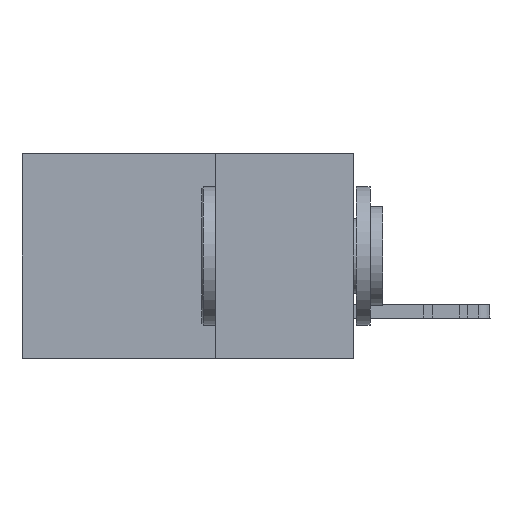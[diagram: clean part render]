
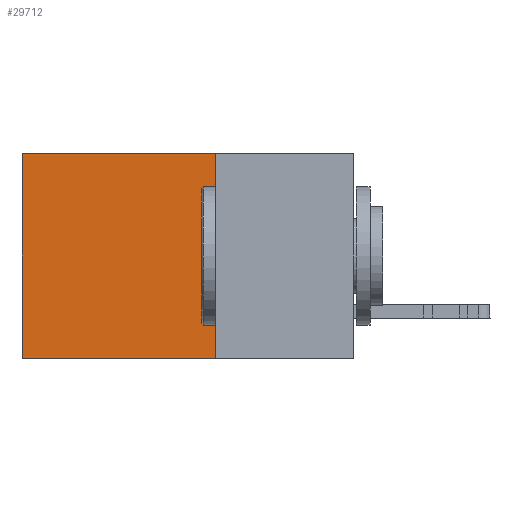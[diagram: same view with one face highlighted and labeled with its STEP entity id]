
A CAD part, left-side view. The second image highlights one B-rep face of the part: STEP entity #29712.
In plain terms, the highlighted planar face has unit normal (-1, 0, 0).
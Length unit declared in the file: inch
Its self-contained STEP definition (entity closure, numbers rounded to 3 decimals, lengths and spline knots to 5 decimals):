
#818 = LINE ( 'NONE', #28860, #31584 ) ;
#3879 = EDGE_CURVE ( 'NONE', #36864, #25628, #8944, .T. ) ;
#6006 = EDGE_CURVE ( 'NONE', #36864, #13630, #818, .T. ) ;
#7831 = DIRECTION ( 'NONE',  ( 0., 0., -1. ) ) ;
#8944 = LINE ( 'NONE', #16353, #35097 ) ;
#9052 = VECTOR ( 'NONE', #17418, 39.37008 ) ;
#10376 = EDGE_LOOP ( 'NONE', ( #10461, #30348, #13086, #15113 ) ) ;
#10461 = ORIENTED_EDGE ( 'NONE', *, *, #25119, .T. ) ;
#11140 = FACE_OUTER_BOUND ( 'NONE', #10376, .T. ) ;
#11546 = LINE ( 'NONE', #42821, #22214 ) ;
#13086 = ORIENTED_EDGE ( 'NONE', *, *, #6006, .F. ) ;
#13630 = VERTEX_POINT ( 'NONE', #16738 ) ;
#14843 = DIRECTION ( 'NONE',  ( 1., 0., 0. ) ) ;
#15113 = ORIENTED_EDGE ( 'NONE', *, *, #3879, .T. ) ;
#15529 = CARTESIAN_POINT ( 'NONE',  ( 0.2875, 0.25, 0. ) ) ;
#16353 = CARTESIAN_POINT ( 'NONE',  ( 0.2875, 0.25, 0. ) ) ;
#16738 = CARTESIAN_POINT ( 'NONE',  ( 0.2875, 0.25, -0.37 ) ) ;
#17418 = DIRECTION ( 'NONE',  ( 0., 1., 0. ) ) ;
#18705 = AXIS2_PLACEMENT_3D ( 'NONE', #39385, #14843, #28955 ) ;
#22214 = VECTOR ( 'NONE', #7831, 39.37008 ) ;
#24355 = LINE ( 'NONE', #31299, #9052 ) ;
#24720 = CARTESIAN_POINT ( 'NONE',  ( 0.2875, 0.6, 0. ) ) ;
#25119 = EDGE_CURVE ( 'NONE', #25628, #35347, #11546, .T. ) ;
#25254 = PLANE ( 'NONE',  #18705 ) ;
#25628 = VERTEX_POINT ( 'NONE', #24720 ) ;
#28860 = CARTESIAN_POINT ( 'NONE',  ( 0.2875, 0.25, 0. ) ) ;
#28955 = DIRECTION ( 'NONE',  ( 0., 0., -1. ) ) ;
#29712 = ADVANCED_FACE ( 'NONE', ( #11140 ), #25254, .F. ) ;
#30348 = ORIENTED_EDGE ( 'NONE', *, *, #36697, .F. ) ;
#30614 = CARTESIAN_POINT ( 'NONE',  ( 0.2875, 0.6, -0.37 ) ) ;
#31299 = CARTESIAN_POINT ( 'NONE',  ( 0.2875, 0.25, -0.37 ) ) ;
#31584 = VECTOR ( 'NONE', #32338, 39.37008 ) ;
#32338 = DIRECTION ( 'NONE',  ( 0., 0., -1. ) ) ;
#35097 = VECTOR ( 'NONE', #37454, 39.37008 ) ;
#35347 = VERTEX_POINT ( 'NONE', #30614 ) ;
#36697 = EDGE_CURVE ( 'NONE', #13630, #35347, #24355, .T. ) ;
#36864 = VERTEX_POINT ( 'NONE', #15529 ) ;
#37454 = DIRECTION ( 'NONE',  ( 0., 1., 0. ) ) ;
#39385 = CARTESIAN_POINT ( 'NONE',  ( 0.2875, 0.25, 0. ) ) ;
#42821 = CARTESIAN_POINT ( 'NONE',  ( 0.2875, 0.6, 0. ) ) ;
